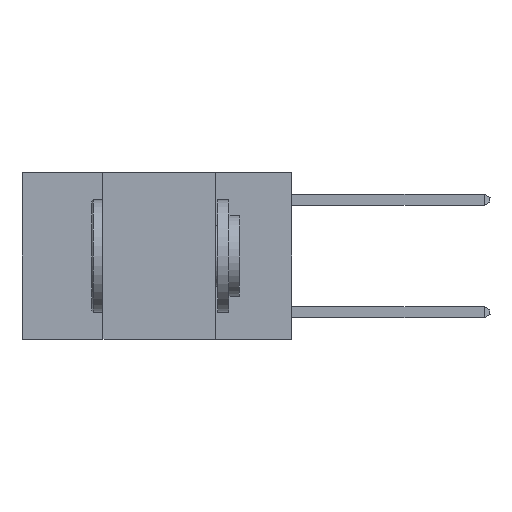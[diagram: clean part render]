
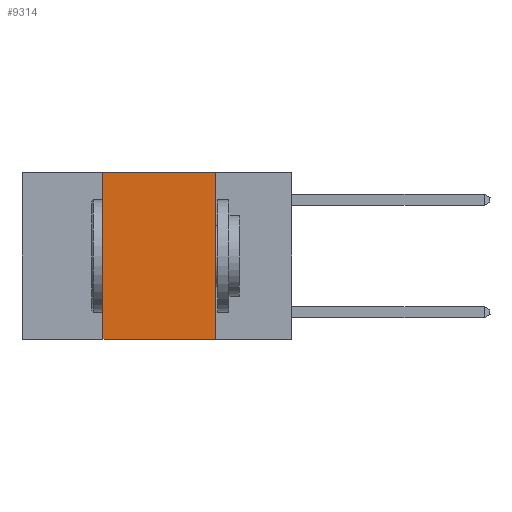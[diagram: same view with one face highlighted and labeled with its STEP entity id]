
A CAD part, left-side view. The second image highlights one B-rep face of the part: STEP entity #9314.
In plain terms, the highlighted planar face has unit normal (-1, 0, 0).
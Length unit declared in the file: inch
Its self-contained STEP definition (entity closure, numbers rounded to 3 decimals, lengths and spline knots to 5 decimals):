
#21 = LINE ( 'NONE', #3433, #6386 ) ;
#703 = LINE ( 'NONE', #12962, #6262 ) ;
#1501 = ORIENTED_EDGE ( 'NONE', *, *, #11825, .F. ) ;
#1615 = DIRECTION ( 'NONE',  ( 0., 0., -1. ) ) ;
#1903 = EDGE_CURVE ( 'NONE', #9527, #2563, #3894, .T. ) ;
#2531 = ORIENTED_EDGE ( 'NONE', *, *, #4144, .T. ) ;
#2563 = VERTEX_POINT ( 'NONE', #5145 ) ;
#2852 = ORIENTED_EDGE ( 'NONE', *, *, #2931, .F. ) ;
#2931 = EDGE_CURVE ( 'NONE', #4032, #8763, #14333, .T. ) ;
#3433 = CARTESIAN_POINT ( 'NONE',  ( 0., 0.6, -0.37 ) ) ;
#3894 = LINE ( 'NONE', #4938, #10854 ) ;
#4032 = VERTEX_POINT ( 'NONE', #5734 ) ;
#4144 = EDGE_CURVE ( 'NONE', #4032, #2563, #21, .T. ) ;
#4146 = CARTESIAN_POINT ( 'NONE',  ( 0., 0.6, 0. ) ) ;
#4938 = CARTESIAN_POINT ( 'NONE',  ( 0., 0.17, 0. ) ) ;
#5145 = CARTESIAN_POINT ( 'NONE',  ( 0., 0.17, -0.37 ) ) ;
#5275 = CARTESIAN_POINT ( 'NONE',  ( 0., 0.42, 0. ) ) ;
#5734 = CARTESIAN_POINT ( 'NONE',  ( 0., 0.42, -0.37 ) ) ;
#5991 = CARTESIAN_POINT ( 'NONE',  ( 0., 0.17, 0. ) ) ;
#6262 = VECTOR ( 'NONE', #8645, 39.37008 ) ;
#6386 = VECTOR ( 'NONE', #7971, 39.37008 ) ;
#7971 = DIRECTION ( 'NONE',  ( 0., -1., 0. ) ) ;
#8645 = DIRECTION ( 'NONE',  ( 0., -1., 0. ) ) ;
#8696 = DIRECTION ( 'NONE',  ( 1., 0., 0. ) ) ;
#8763 = VERTEX_POINT ( 'NONE', #9816 ) ;
#9314 = ADVANCED_FACE ( 'NONE', ( #9793 ), #14323, .F. ) ;
#9527 = VERTEX_POINT ( 'NONE', #5991 ) ;
#9545 = EDGE_LOOP ( 'NONE', ( #11115, #1501, #2852, #2531 ) ) ;
#9584 = DIRECTION ( 'NONE',  ( 0., 0., 1. ) ) ;
#9793 = FACE_OUTER_BOUND ( 'NONE', #9545, .T. ) ;
#9816 = CARTESIAN_POINT ( 'NONE',  ( 0., 0.42, 0. ) ) ;
#10854 = VECTOR ( 'NONE', #1615, 39.37008 ) ;
#11009 = DIRECTION ( 'NONE',  ( 0., 0., -1. ) ) ;
#11115 = ORIENTED_EDGE ( 'NONE', *, *, #1903, .F. ) ;
#11825 = EDGE_CURVE ( 'NONE', #8763, #9527, #703, .T. ) ;
#12962 = CARTESIAN_POINT ( 'NONE',  ( 0., 0.6, 0. ) ) ;
#13049 = VECTOR ( 'NONE', #9584, 39.37008 ) ;
#13805 = AXIS2_PLACEMENT_3D ( 'NONE', #4146, #8696, #11009 ) ;
#14323 = PLANE ( 'NONE',  #13805 ) ;
#14333 = LINE ( 'NONE', #5275, #13049 ) ;
